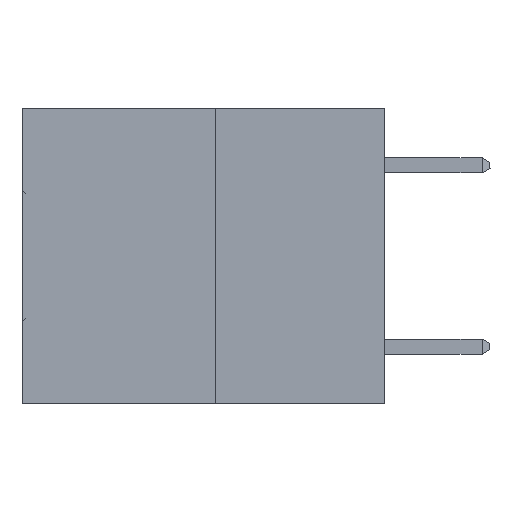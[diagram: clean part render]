
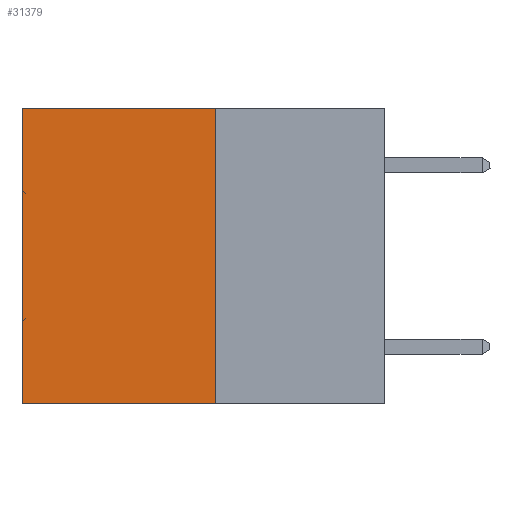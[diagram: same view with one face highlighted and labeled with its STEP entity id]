
A CAD part, left-side view. The second image highlights one B-rep face of the part: STEP entity #31379.
In plain terms, the highlighted planar face has unit normal (-1, 0, 0).
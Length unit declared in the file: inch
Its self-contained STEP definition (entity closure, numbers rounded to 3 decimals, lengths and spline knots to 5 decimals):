
#2146 = DIRECTION ( 'NONE',  ( 0., 0., -1. ) ) ;
#3848 = ORIENTED_EDGE ( 'NONE', *, *, #19195, .T. ) ;
#4025 = PLANE ( 'NONE',  #34559 ) ;
#5189 = CARTESIAN_POINT ( 'NONE',  ( 0.3165, 0.6, 0. ) ) ;
#8739 = LINE ( 'NONE', #14552, #17293 ) ;
#8848 = VERTEX_POINT ( 'NONE', #15532 ) ;
#10708 = VERTEX_POINT ( 'NONE', #15246 ) ;
#11558 = LINE ( 'NONE', #27819, #12806 ) ;
#11971 = VECTOR ( 'NONE', #25679, 39.37008 ) ;
#12407 = EDGE_CURVE ( 'NONE', #8848, #24761, #8739, .T. ) ;
#12806 = VECTOR ( 'NONE', #30404, 39.37008 ) ;
#13047 = CARTESIAN_POINT ( 'NONE',  ( 0.3165, 0.6, -0.49 ) ) ;
#14552 = CARTESIAN_POINT ( 'NONE',  ( 0.3165, 0.28, 0. ) ) ;
#15223 = EDGE_CURVE ( 'NONE', #8848, #21440, #11558, .T. ) ;
#15246 = CARTESIAN_POINT ( 'NONE',  ( 0.3165, 0.6, -0.49 ) ) ;
#15532 = CARTESIAN_POINT ( 'NONE',  ( 0.3165, 0.28, 0. ) ) ;
#16383 = ORIENTED_EDGE ( 'NONE', *, *, #12407, .T. ) ;
#16854 = ORIENTED_EDGE ( 'NONE', *, *, #15223, .F. ) ;
#17293 = VECTOR ( 'NONE', #22995, 39.37008 ) ;
#17753 = CARTESIAN_POINT ( 'NONE',  ( 0.3165, 0.28, -0.49 ) ) ;
#18470 = EDGE_CURVE ( 'NONE', #21440, #10708, #29319, .T. ) ;
#19195 = EDGE_CURVE ( 'NONE', #24761, #10708, #24840, .T. ) ;
#20048 = EDGE_LOOP ( 'NONE', ( #3848, #35753, #16854, #16383 ) ) ;
#21440 = VERTEX_POINT ( 'NONE', #17753 ) ;
#22995 = DIRECTION ( 'NONE',  ( 0., 1., 0. ) ) ;
#24761 = VERTEX_POINT ( 'NONE', #5189 ) ;
#24840 = LINE ( 'NONE', #13047, #32654 ) ;
#25679 = DIRECTION ( 'NONE',  ( 0., 1., 0. ) ) ;
#27819 = CARTESIAN_POINT ( 'NONE',  ( 0.3165, 0.28, -0.49 ) ) ;
#28864 = FACE_OUTER_BOUND ( 'NONE', #20048, .T. ) ;
#29171 = CARTESIAN_POINT ( 'NONE',  ( 0.3165, 0.28, -0.49 ) ) ;
#29319 = LINE ( 'NONE', #31204, #11971 ) ;
#30404 = DIRECTION ( 'NONE',  ( 0., 0., -1. ) ) ;
#31204 = CARTESIAN_POINT ( 'NONE',  ( 0.3165, 0.28, -0.49 ) ) ;
#31379 = ADVANCED_FACE ( 'NONE', ( #28864 ), #4025, .F. ) ;
#31714 = DIRECTION ( 'NONE',  ( 1., 0., 0. ) ) ;
#32654 = VECTOR ( 'NONE', #2146, 39.37008 ) ;
#34460 = DIRECTION ( 'NONE',  ( 0., 0., -1. ) ) ;
#34559 = AXIS2_PLACEMENT_3D ( 'NONE', #29171, #31714, #34460 ) ;
#35753 = ORIENTED_EDGE ( 'NONE', *, *, #18470, .F. ) ;
